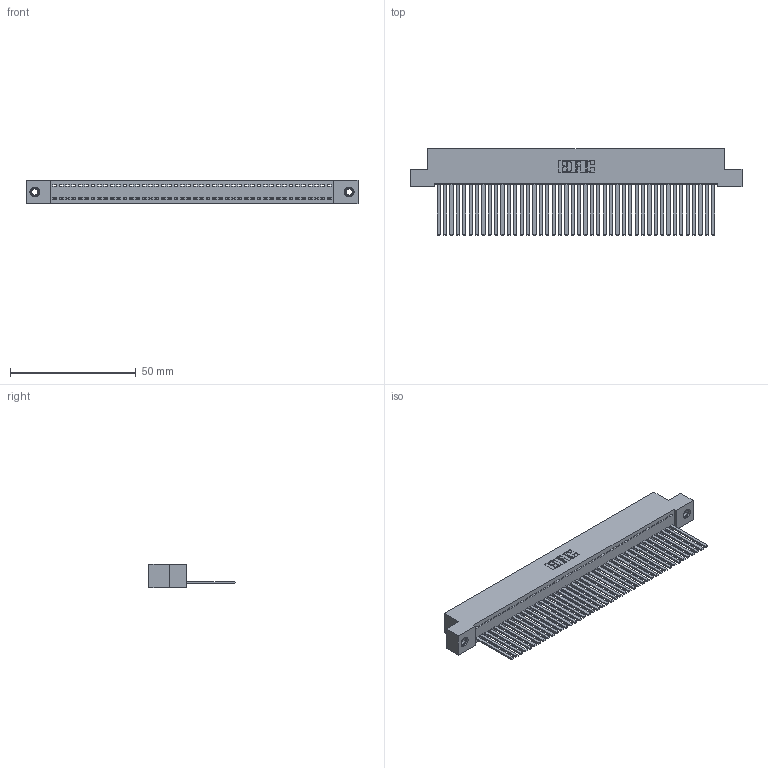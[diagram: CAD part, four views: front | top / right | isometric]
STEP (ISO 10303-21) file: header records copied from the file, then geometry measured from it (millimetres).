
FILE_DESCRIPTION (( 'STEP AP203' ), '1' );
FILE_NAME ('392-044-544-107.STEP', '2018-08-16T15:23:47', ( '' ), ( '' ), 'SwSTEP 2.0', 'SolidWorks 2016', '' );
FILE_SCHEMA (( 'CONFIG_CONTROL_DESIGN' ));
Length unit declared in the file: inch
Products named in the file (4): 345-250-001_345-250-005-103; 392-044-544-107; 342 Part_TI; 345-292-001_345-293-144
Assembly tree (47 placements, depth 2):
  392-044-544-107
    342 Part_TI
    345-292-001_345-293-144  x44
    345-250-001_345-250-005-103  x2
Bounding box: 132.08 x 34.3 x 9.4 mm (x, y, z)
Volume: 12085 mm3; surface area: 19266.2 mm2
Topology: 47 solids, 47 shells, 2458 faces, 7387 edges, 4858 vertices
Faces by surface type: plane 1770, cylinder 672, cone 12, torus 4
Entity records: 27510 total; most frequent: CARTESIAN_POINT 4725, ORIENTED_EDGE 4698, DIRECTION 4011, EDGE_CURVE 2349, VECTOR 2205, LINE 2205, VERTEX_POINT 1560, AXIS2_PLACEMENT_3D 903
